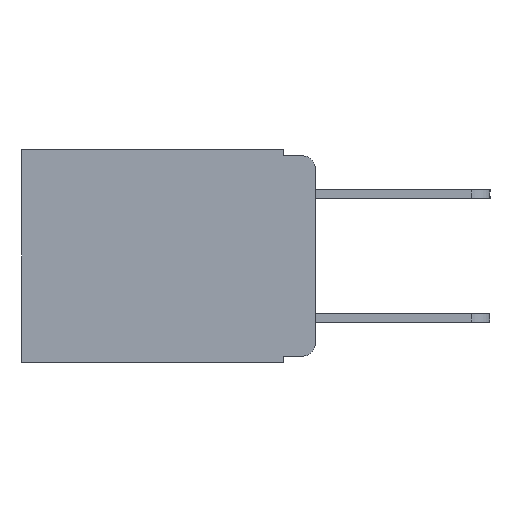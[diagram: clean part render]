
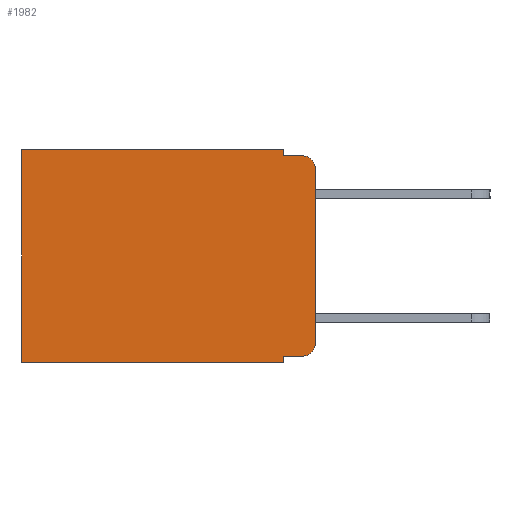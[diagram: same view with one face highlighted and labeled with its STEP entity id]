
A CAD part, left-side view. The second image highlights one B-rep face of the part: STEP entity #1982.
In plain terms, the highlighted planar face has unit normal (-1, 0, 0).
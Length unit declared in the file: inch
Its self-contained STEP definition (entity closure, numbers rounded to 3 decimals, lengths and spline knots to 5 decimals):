
#299 = ORIENTED_EDGE ( 'NONE', *, *, #12356, .F. ) ;
#331 = ORIENTED_EDGE ( 'NONE', *, *, #3416, .F. ) ;
#473 = VERTEX_POINT ( 'NONE', #10138 ) ;
#723 = VERTEX_POINT ( 'NONE', #7360 ) ;
#761 = AXIS2_PLACEMENT_3D ( 'NONE', #15896, #8002, #9629 ) ;
#894 = CARTESIAN_POINT ( 'NONE',  ( 0.298, 0.051, -0.333 ) ) ;
#1912 = DIRECTION ( 'NONE',  ( 0., 0., -1. ) ) ;
#1917 = ORIENTED_EDGE ( 'NONE', *, *, #15377, .F. ) ;
#1982 = ADVANCED_FACE ( 'NONE', ( #5872 ), #16404, .F. ) ;
#2003 = CARTESIAN_POINT ( 'NONE',  ( 0.298, 0.473, -0.343 ) ) ;
#2179 = VERTEX_POINT ( 'NONE', #9512 ) ;
#2782 = CARTESIAN_POINT ( 'NONE',  ( 0.298, 0.051, 0. ) ) ;
#2917 = LINE ( 'NONE', #17459, #19886 ) ;
#3145 = VERTEX_POINT ( 'NONE', #2003 ) ;
#3362 = CIRCLE ( 'NONE', #761, 0.02 ) ;
#3416 = EDGE_CURVE ( 'NONE', #15105, #21157, #8158, .T. ) ;
#4080 = CARTESIAN_POINT ( 'NONE',  ( 0.298, 0.473, 0. ) ) ;
#5232 = AXIS2_PLACEMENT_3D ( 'NONE', #8681, #12380, #7392 ) ;
#5308 = CARTESIAN_POINT ( 'NONE',  ( 0.298, 0.051, -0.01 ) ) ;
#5872 = FACE_OUTER_BOUND ( 'NONE', #15194, .T. ) ;
#6309 = EDGE_CURVE ( 'NONE', #19318, #21157, #3362, .T. ) ;
#7079 = CARTESIAN_POINT ( 'NONE',  ( 0.298, 0.051, -0.01 ) ) ;
#7360 = CARTESIAN_POINT ( 'NONE',  ( 0.298, 0., -0.313 ) ) ;
#7392 = DIRECTION ( 'NONE',  ( 0., 0., -1. ) ) ;
#7399 = LINE ( 'NONE', #16849, #19965 ) ;
#7736 = VECTOR ( 'NONE', #1912, 39.37008 ) ;
#7933 = ORIENTED_EDGE ( 'NONE', *, *, #6309, .T. ) ;
#8002 = DIRECTION ( 'NONE',  ( -1., 0., 0. ) ) ;
#8090 = VECTOR ( 'NONE', #15130, 39.37008 ) ;
#8158 = LINE ( 'NONE', #7079, #16353 ) ;
#8282 = CARTESIAN_POINT ( 'NONE',  ( 0.298, 0., 0. ) ) ;
#8444 = CARTESIAN_POINT ( 'NONE',  ( 0.298, 0.02, -0.313 ) ) ;
#8460 = ORIENTED_EDGE ( 'NONE', *, *, #8919, .T. ) ;
#8681 = CARTESIAN_POINT ( 'NONE',  ( 0.298, 0., 0. ) ) ;
#8919 = EDGE_CURVE ( 'NONE', #2179, #19674, #11329, .T. ) ;
#8932 = ORIENTED_EDGE ( 'NONE', *, *, #11089, .F. ) ;
#9044 = EDGE_CURVE ( 'NONE', #19318, #723, #20817, .T. ) ;
#9167 = EDGE_CURVE ( 'NONE', #11877, #723, #14402, .T. ) ;
#9369 = VECTOR ( 'NONE', #14306, 39.37008 ) ;
#9512 = CARTESIAN_POINT ( 'NONE',  ( 0.298, 0.051, 0. ) ) ;
#9629 = DIRECTION ( 'NONE',  ( 0., 0., -1. ) ) ;
#9910 = DIRECTION ( 'NONE',  ( 0., 1., 0. ) ) ;
#10067 = DIRECTION ( 'NONE',  ( 0., 0., -1. ) ) ;
#10138 = CARTESIAN_POINT ( 'NONE',  ( 0.298, 0.051, -0.343 ) ) ;
#10331 = AXIS2_PLACEMENT_3D ( 'NONE', #8444, #19927, #10067 ) ;
#10561 = EDGE_CURVE ( 'NONE', #19674, #3145, #17172, .T. ) ;
#11089 = EDGE_CURVE ( 'NONE', #473, #3145, #7399, .T. ) ;
#11329 = LINE ( 'NONE', #8282, #19056 ) ;
#11877 = VERTEX_POINT ( 'NONE', #13948 ) ;
#12356 = EDGE_CURVE ( 'NONE', #2179, #15105, #13747, .T. ) ;
#12380 = DIRECTION ( 'NONE',  ( 1., 0., 0. ) ) ;
#12568 = DIRECTION ( 'NONE',  ( 0., 0., -1. ) ) ;
#12810 = VECTOR ( 'NONE', #18894, 39.37008 ) ;
#13747 = LINE ( 'NONE', #2782, #9369 ) ;
#13768 = ORIENTED_EDGE ( 'NONE', *, *, #9044, .F. ) ;
#13948 = CARTESIAN_POINT ( 'NONE',  ( 0.298, 0.02, -0.333 ) ) ;
#14306 = DIRECTION ( 'NONE',  ( 0., 0., -1. ) ) ;
#14402 = CIRCLE ( 'NONE', #10331, 0.02 ) ;
#15035 = CARTESIAN_POINT ( 'NONE',  ( 0.298, 0.02, -0.01 ) ) ;
#15094 = CARTESIAN_POINT ( 'NONE',  ( 0.298, 0., 0. ) ) ;
#15105 = VERTEX_POINT ( 'NONE', #5308 ) ;
#15130 = DIRECTION ( 'NONE',  ( 0., -1., 0. ) ) ;
#15194 = EDGE_LOOP ( 'NONE', ( #13768, #7933, #331, #299, #8460, #19392, #8932, #1917, #20290, #16135 ) ) ;
#15377 = EDGE_CURVE ( 'NONE', #17171, #473, #2917, .T. ) ;
#15877 = CARTESIAN_POINT ( 'NONE',  ( 0.298, 0., -0.03 ) ) ;
#15896 = CARTESIAN_POINT ( 'NONE',  ( 0.298, 0.02, -0.03 ) ) ;
#16135 = ORIENTED_EDGE ( 'NONE', *, *, #9167, .T. ) ;
#16353 = VECTOR ( 'NONE', #19604, 39.37008 ) ;
#16404 = PLANE ( 'NONE',  #5232 ) ;
#16777 = CARTESIAN_POINT ( 'NONE',  ( 0.298, 0.051, -0.333 ) ) ;
#16849 = CARTESIAN_POINT ( 'NONE',  ( 0.298, 0., -0.343 ) ) ;
#17171 = VERTEX_POINT ( 'NONE', #894 ) ;
#17172 = LINE ( 'NONE', #4080, #12810 ) ;
#17459 = CARTESIAN_POINT ( 'NONE',  ( 0.298, 0.051, 0. ) ) ;
#18511 = DIRECTION ( 'NONE',  ( 0., 1., 0. ) ) ;
#18894 = DIRECTION ( 'NONE',  ( 0., 0., -1. ) ) ;
#19056 = VECTOR ( 'NONE', #9910, 39.37008 ) ;
#19318 = VERTEX_POINT ( 'NONE', #15877 ) ;
#19392 = ORIENTED_EDGE ( 'NONE', *, *, #10561, .T. ) ;
#19604 = DIRECTION ( 'NONE',  ( 0., -1., 0. ) ) ;
#19674 = VERTEX_POINT ( 'NONE', #20083 ) ;
#19886 = VECTOR ( 'NONE', #12568, 39.37008 ) ;
#19927 = DIRECTION ( 'NONE',  ( -1., 0., 0. ) ) ;
#19965 = VECTOR ( 'NONE', #18511, 39.37008 ) ;
#20083 = CARTESIAN_POINT ( 'NONE',  ( 0.298, 0.473, 0. ) ) ;
#20175 = EDGE_CURVE ( 'NONE', #17171, #11877, #21156, .T. ) ;
#20290 = ORIENTED_EDGE ( 'NONE', *, *, #20175, .T. ) ;
#20817 = LINE ( 'NONE', #15094, #7736 ) ;
#21156 = LINE ( 'NONE', #16777, #8090 ) ;
#21157 = VERTEX_POINT ( 'NONE', #15035 ) ;
